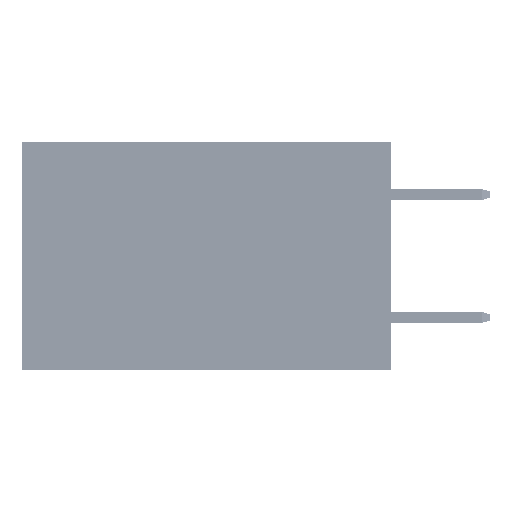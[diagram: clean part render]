
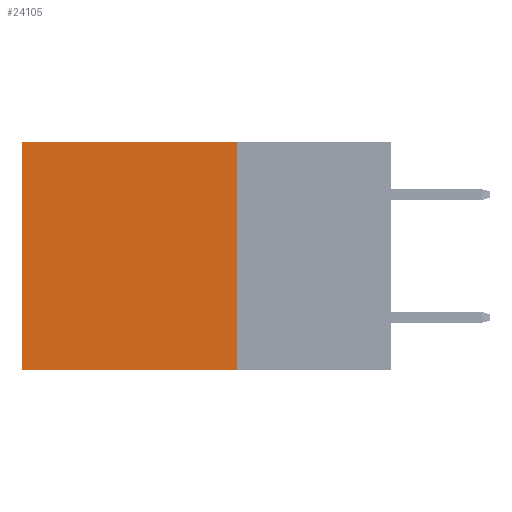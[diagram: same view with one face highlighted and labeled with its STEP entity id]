
A CAD part, left-side view. The second image highlights one B-rep face of the part: STEP entity #24105.
In plain terms, the highlighted planar face has unit normal (-1, 0, 0).
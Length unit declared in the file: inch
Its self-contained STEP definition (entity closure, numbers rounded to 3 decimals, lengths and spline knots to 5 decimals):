
#2866 = VECTOR ( 'NONE', #4449, 39.37008 ) ;
#4009 = VECTOR ( 'NONE', #25531, 39.37008 ) ;
#4449 = DIRECTION ( 'NONE',  ( 0., 0., -1. ) ) ;
#6380 = EDGE_CURVE ( 'NONE', #23161, #29926, #29571, .T. ) ;
#7435 = DIRECTION ( 'NONE',  ( 1., 0., 0. ) ) ;
#7767 = ORIENTED_EDGE ( 'NONE', *, *, #33111, .F. ) ;
#8369 = CARTESIAN_POINT ( 'NONE',  ( 0.2875, 0.25, 0. ) ) ;
#10274 = VECTOR ( 'NONE', #30956, 39.37008 ) ;
#10356 = ORIENTED_EDGE ( 'NONE', *, *, #20662, .T. ) ;
#11246 = FACE_OUTER_BOUND ( 'NONE', #25748, .T. ) ;
#13627 = DIRECTION ( 'NONE',  ( 0., 1., 0. ) ) ;
#14046 = ORIENTED_EDGE ( 'NONE', *, *, #46994, .T. ) ;
#17003 = CARTESIAN_POINT ( 'NONE',  ( 0.2875, 0.25, -0.37 ) ) ;
#17207 = CARTESIAN_POINT ( 'NONE',  ( 0.2875, 0.25, -0.37 ) ) ;
#19894 = AXIS2_PLACEMENT_3D ( 'NONE', #8369, #7435, #22206 ) ;
#19949 = CARTESIAN_POINT ( 'NONE',  ( 0.2875, 0.25, 0. ) ) ;
#20662 = EDGE_CURVE ( 'NONE', #37587, #46288, #23024, .T. ) ;
#22206 = DIRECTION ( 'NONE',  ( 0., 0., -1. ) ) ;
#23024 = LINE ( 'NONE', #25663, #2866 ) ;
#23161 = VERTEX_POINT ( 'NONE', #39360 ) ;
#24105 = ADVANCED_FACE ( 'NONE', ( #11246 ), #44175, .F. ) ;
#24127 = LINE ( 'NONE', #17207, #24205 ) ;
#24205 = VECTOR ( 'NONE', #13627, 39.37008 ) ;
#25531 = DIRECTION ( 'NONE',  ( 0., 0., -1. ) ) ;
#25663 = CARTESIAN_POINT ( 'NONE',  ( 0.2875, 0.6, 0. ) ) ;
#25748 = EDGE_LOOP ( 'NONE', ( #10356, #7767, #28623, #14046 ) ) ;
#28623 = ORIENTED_EDGE ( 'NONE', *, *, #6380, .F. ) ;
#29116 = CARTESIAN_POINT ( 'NONE',  ( 0.2875, 0.6, -0.37 ) ) ;
#29571 = LINE ( 'NONE', #44846, #4009 ) ;
#29926 = VERTEX_POINT ( 'NONE', #17003 ) ;
#30956 = DIRECTION ( 'NONE',  ( 0., 1., 0. ) ) ;
#33111 = EDGE_CURVE ( 'NONE', #29926, #46288, #24127, .T. ) ;
#37587 = VERTEX_POINT ( 'NONE', #39801 ) ;
#39360 = CARTESIAN_POINT ( 'NONE',  ( 0.2875, 0.25, 0. ) ) ;
#39801 = CARTESIAN_POINT ( 'NONE',  ( 0.2875, 0.6, 0. ) ) ;
#44175 = PLANE ( 'NONE',  #19894 ) ;
#44846 = CARTESIAN_POINT ( 'NONE',  ( 0.2875, 0.25, 0. ) ) ;
#46223 = LINE ( 'NONE', #19949, #10274 ) ;
#46288 = VERTEX_POINT ( 'NONE', #29116 ) ;
#46994 = EDGE_CURVE ( 'NONE', #23161, #37587, #46223, .T. ) ;
